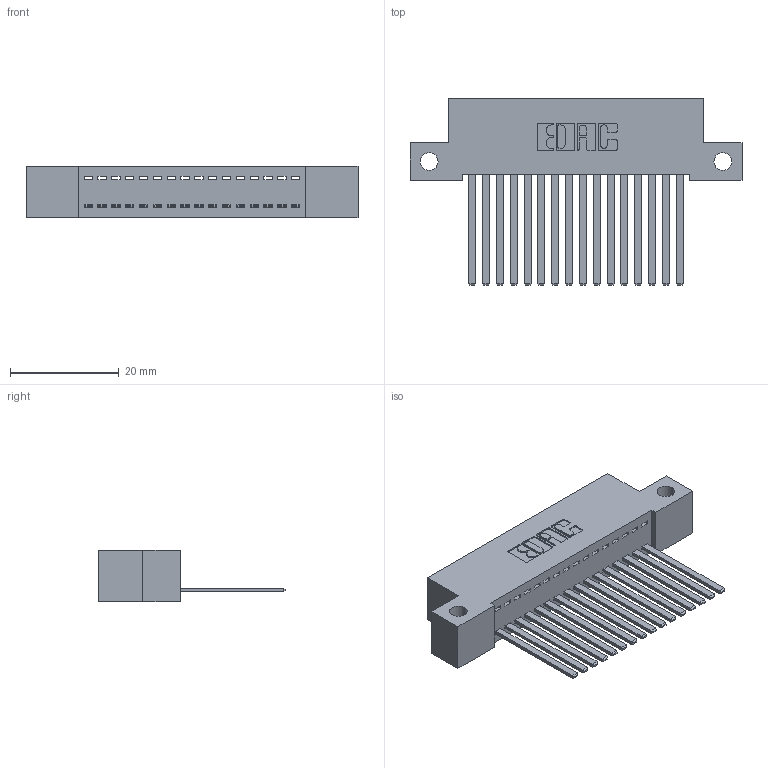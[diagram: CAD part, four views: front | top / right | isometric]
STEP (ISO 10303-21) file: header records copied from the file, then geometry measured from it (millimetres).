
FILE_DESCRIPTION (( 'STEP AP203' ), '1' );
FILE_NAME ('392-016-544-112.STEP', '2019-10-07T03:19:24', ( '' ), ( '' ), 'SwSTEP 2.0', 'SolidWorks 2016', '' );
FILE_SCHEMA (( 'CONFIG_CONTROL_DESIGN' ));
Length unit declared in the file: inch
Products named in the file (3): 342 Part_Side Mount; 345-292-001_345-293-144; 392-016-544-112
Assembly tree (17 placements, depth 2):
  392-016-544-112
    342 Part_Side Mount
    345-292-001_345-293-144  x16
Bounding box: 60.96 x 34.3 x 9.4 mm (x, y, z)
Volume: 5360.6 mm3; surface area: 7750.6 mm2
Topology: 17 solids, 17 shells, 942 faces, 2827 edges, 1862 vertices
Faces by surface type: plane 674, cylinder 268
Entity records: 12831 total; most frequent: CARTESIAN_POINT 2222, ORIENTED_EDGE 2174, DIRECTION 1923, EDGE_CURVE 1087, LINE 963, VECTOR 963, VERTEX_POINT 722, AXIS2_PLACEMENT_3D 480
